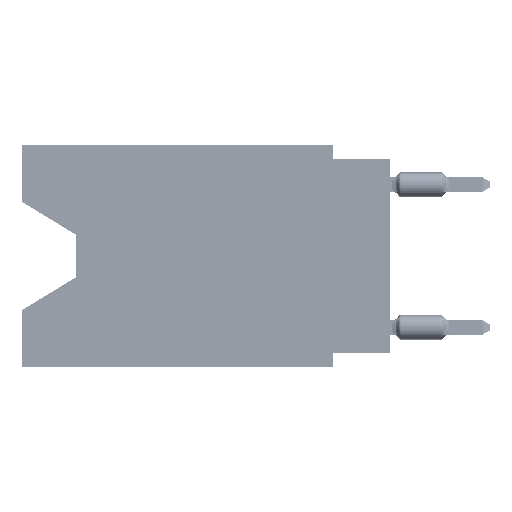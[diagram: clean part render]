
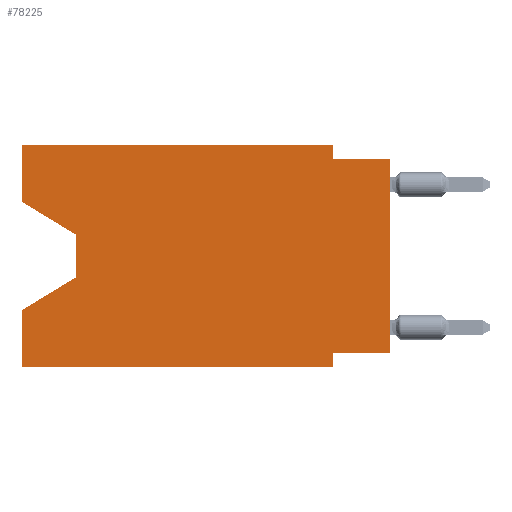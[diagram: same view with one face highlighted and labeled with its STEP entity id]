
A CAD part, left-side view. The second image highlights one B-rep face of the part: STEP entity #78225.
In plain terms, the highlighted planar face has unit normal (-1, 0, 0).
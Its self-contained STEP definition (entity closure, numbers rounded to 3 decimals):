
#139 = CARTESIAN_POINT ( 'NONE',  ( 0., 16.383, -9.906 ) ) ;
#903 = AXIS2_PLACEMENT_3D ( 'NONE', #10982, #3018, #35388 ) ;
#2113 = ORIENTED_EDGE ( 'NONE', *, *, #82697, .F. ) ;
#2192 = LINE ( 'NONE', #77858, #24596 ) ;
#3018 = DIRECTION ( 'NONE',  ( 1., 0., 0. ) ) ;
#4289 = ORIENTED_EDGE ( 'NONE', *, *, #56455, .T. ) ;
#5489 = CARTESIAN_POINT ( 'NONE',  ( 0., 0., -0.635 ) ) ;
#5551 = ORIENTED_EDGE ( 'NONE', *, *, #34573, .T. ) ;
#6151 = CARTESIAN_POINT ( 'NONE',  ( 0., 13.97, -5.893 ) ) ;
#9471 = CARTESIAN_POINT ( 'NONE',  ( 0., 2.54, -0.635 ) ) ;
#10982 = CARTESIAN_POINT ( 'NONE',  ( 0., 16.383, 0. ) ) ;
#13940 = VERTEX_POINT ( 'NONE', #46910 ) ;
#14719 = ORIENTED_EDGE ( 'NONE', *, *, #76071, .T. ) ;
#17060 = CARTESIAN_POINT ( 'NONE',  ( 0., 13.97, -4.013 ) ) ;
#17283 = CARTESIAN_POINT ( 'NONE',  ( 0., 13.97, -4.013 ) ) ;
#17482 = DIRECTION ( 'NONE',  ( 0., 0., 1. ) ) ;
#17708 = CARTESIAN_POINT ( 'NONE',  ( 0., 16.383, -2.546 ) ) ;
#18304 = LINE ( 'NONE', #37225, #60020 ) ;
#18410 = CARTESIAN_POINT ( 'NONE',  ( 0., 2.54, 0. ) ) ;
#19611 = VERTEX_POINT ( 'NONE', #6151 ) ;
#19614 = EDGE_CURVE ( 'NONE', #68079, #26244, #31794, .T. ) ;
#20011 = DIRECTION ( 'NONE',  ( 0., -1., 0. ) ) ;
#21165 = ORIENTED_EDGE ( 'NONE', *, *, #45809, .T. ) ;
#21286 = LINE ( 'NONE', #40215, #27717 ) ;
#24596 = VECTOR ( 'NONE', #28238, 1000. ) ;
#24604 = CARTESIAN_POINT ( 'NONE',  ( 0., 13.97, -5.893 ) ) ;
#26244 = VERTEX_POINT ( 'NONE', #27612 ) ;
#27612 = CARTESIAN_POINT ( 'NONE',  ( 0., 2.54, 0. ) ) ;
#27691 = CARTESIAN_POINT ( 'NONE',  ( 0., 16.383, -2.546 ) ) ;
#27717 = VECTOR ( 'NONE', #46922, 1000. ) ;
#28238 = DIRECTION ( 'NONE',  ( 0., -1., 0. ) ) ;
#28658 = PLANE ( 'NONE',  #903 ) ;
#29206 = CARTESIAN_POINT ( 'NONE',  ( 0., 16.383, 0. ) ) ;
#30313 = LINE ( 'NONE', #61815, #66330 ) ;
#30424 = CARTESIAN_POINT ( 'NONE',  ( 0., 0., -9.271 ) ) ;
#30678 = VERTEX_POINT ( 'NONE', #69774 ) ;
#31794 = LINE ( 'NONE', #83039, #58259 ) ;
#31796 = VECTOR ( 'NONE', #77598, 1000. ) ;
#32023 = VECTOR ( 'NONE', #43346, 1000. ) ;
#33342 = VERTEX_POINT ( 'NONE', #17060 ) ;
#34573 = EDGE_CURVE ( 'NONE', #19611, #46511, #43551, .T. ) ;
#35388 = DIRECTION ( 'NONE',  ( 0., 0., -1. ) ) ;
#36065 = VERTEX_POINT ( 'NONE', #80863 ) ;
#36460 = ORIENTED_EDGE ( 'NONE', *, *, #81556, .F. ) ;
#36582 = VERTEX_POINT ( 'NONE', #17708 ) ;
#36633 = FACE_OUTER_BOUND ( 'NONE', #47939, .T. ) ;
#36923 = LINE ( 'NONE', #18410, #79238 ) ;
#37225 = CARTESIAN_POINT ( 'NONE',  ( 0., 16.383, 0. ) ) ;
#37650 = EDGE_CURVE ( 'NONE', #36582, #68079, #18304, .T. ) ;
#38490 = EDGE_CURVE ( 'NONE', #53427, #13940, #55937, .T. ) ;
#39377 = VECTOR ( 'NONE', #67826, 1000. ) ;
#40215 = CARTESIAN_POINT ( 'NONE',  ( 0., 0., 0. ) ) ;
#42629 = CARTESIAN_POINT ( 'NONE',  ( 0., 2.54, -9.271 ) ) ;
#43346 = DIRECTION ( 'NONE',  ( 0., -1., 0. ) ) ;
#43551 = LINE ( 'NONE', #24604, #69847 ) ;
#45809 = EDGE_CURVE ( 'NONE', #33342, #19611, #74839, .T. ) ;
#46511 = VERTEX_POINT ( 'NONE', #59957 ) ;
#46910 = CARTESIAN_POINT ( 'NONE',  ( 0., 0., -0.635 ) ) ;
#46922 = DIRECTION ( 'NONE',  ( 0., 0., 1. ) ) ;
#47939 = EDGE_LOOP ( 'NONE', ( #4289, #21165, #5551, #2113, #75215, #71467, #36460, #14719, #58972, #68986, #53329, #57139 ) ) ;
#49904 = VERTEX_POINT ( 'NONE', #42629 ) ;
#51971 = CARTESIAN_POINT ( 'NONE',  ( 0., 2.54, -9.906 ) ) ;
#53329 = ORIENTED_EDGE ( 'NONE', *, *, #19614, .F. ) ;
#53330 = DIRECTION ( 'NONE',  ( 0., -0.855, -0.519 ) ) ;
#53427 = VERTEX_POINT ( 'NONE', #9471 ) ;
#54602 = EDGE_CURVE ( 'NONE', #49904, #30678, #58255, .T. ) ;
#55937 = LINE ( 'NONE', #5489, #32023 ) ;
#56046 = LINE ( 'NONE', #30424, #39377 ) ;
#56455 = EDGE_CURVE ( 'NONE', #36582, #33342, #72638, .T. ) ;
#57139 = ORIENTED_EDGE ( 'NONE', *, *, #37650, .F. ) ;
#58255 = LINE ( 'NONE', #51971, #31796 ) ;
#58259 = VECTOR ( 'NONE', #20011, 1000. ) ;
#58972 = ORIENTED_EDGE ( 'NONE', *, *, #38490, .F. ) ;
#59957 = CARTESIAN_POINT ( 'NONE',  ( 0., 16.383, -7.36 ) ) ;
#60020 = VECTOR ( 'NONE', #17482, 1000. ) ;
#61815 = CARTESIAN_POINT ( 'NONE',  ( 0., 16.383, 0. ) ) ;
#62536 = DIRECTION ( 'NONE',  ( 0., 0., -1. ) ) ;
#62788 = EDGE_CURVE ( 'NONE', #72908, #30678, #2192, .T. ) ;
#66266 = VECTOR ( 'NONE', #68541, 1000. ) ;
#66330 = VECTOR ( 'NONE', #81989, 1000. ) ;
#67826 = DIRECTION ( 'NONE',  ( 0., 1., 0. ) ) ;
#68079 = VERTEX_POINT ( 'NONE', #29206 ) ;
#68541 = DIRECTION ( 'NONE',  ( 0., 0., -1. ) ) ;
#68739 = DIRECTION ( 'NONE',  ( 0., 0.855, -0.519 ) ) ;
#68986 = ORIENTED_EDGE ( 'NONE', *, *, #70740, .F. ) ;
#69774 = CARTESIAN_POINT ( 'NONE',  ( 0., 2.54, -9.906 ) ) ;
#69847 = VECTOR ( 'NONE', #68739, 1000. ) ;
#70647 = VECTOR ( 'NONE', #53330, 1000. ) ;
#70740 = EDGE_CURVE ( 'NONE', #26244, #53427, #36923, .T. ) ;
#71467 = ORIENTED_EDGE ( 'NONE', *, *, #54602, .F. ) ;
#72638 = LINE ( 'NONE', #27691, #70647 ) ;
#72908 = VERTEX_POINT ( 'NONE', #139 ) ;
#74839 = LINE ( 'NONE', #17283, #66266 ) ;
#75215 = ORIENTED_EDGE ( 'NONE', *, *, #62788, .T. ) ;
#76071 = EDGE_CURVE ( 'NONE', #36065, #13940, #21286, .T. ) ;
#77598 = DIRECTION ( 'NONE',  ( 0., 0., -1. ) ) ;
#77858 = CARTESIAN_POINT ( 'NONE',  ( 0., 16.383, -9.906 ) ) ;
#78225 = ADVANCED_FACE ( 'NONE', ( #36633 ), #28658, .F. ) ;
#79238 = VECTOR ( 'NONE', #62536, 1000. ) ;
#80863 = CARTESIAN_POINT ( 'NONE',  ( 0., 0., -9.271 ) ) ;
#81556 = EDGE_CURVE ( 'NONE', #36065, #49904, #56046, .T. ) ;
#81989 = DIRECTION ( 'NONE',  ( 0., 0., 1. ) ) ;
#82697 = EDGE_CURVE ( 'NONE', #72908, #46511, #30313, .T. ) ;
#83039 = CARTESIAN_POINT ( 'NONE',  ( 0., 16.383, 0. ) ) ;
